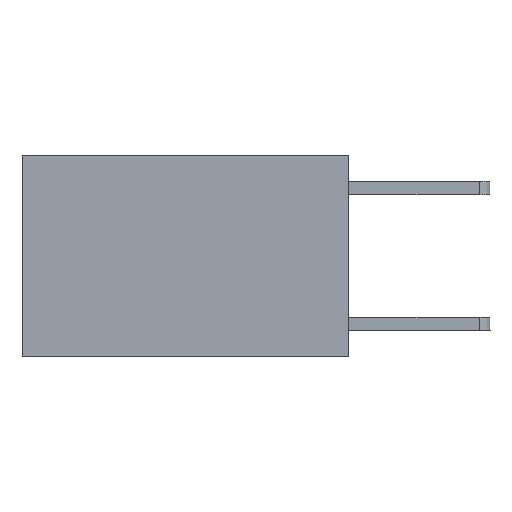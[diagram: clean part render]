
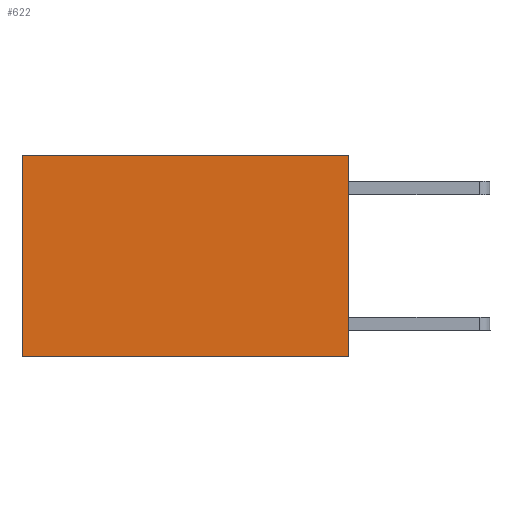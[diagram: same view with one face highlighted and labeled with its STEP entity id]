
A CAD part, left-side view. The second image highlights one B-rep face of the part: STEP entity #622.
In plain terms, the highlighted planar face has unit normal (-1, 0, 0).
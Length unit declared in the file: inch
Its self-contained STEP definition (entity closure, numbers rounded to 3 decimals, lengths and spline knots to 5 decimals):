
#97 = CARTESIAN_POINT ( 'NONE',  ( 0.2625, 0.6, -0.37 ) ) ;
#622 = ADVANCED_FACE ( 'NONE', ( #1866 ), #4625, .F. ) ;
#1021 = LINE ( 'NONE', #7380, #8252 ) ;
#1254 = VECTOR ( 'NONE', #7338, 39.37008 ) ;
#1770 = ORIENTED_EDGE ( 'NONE', *, *, #6092, .T. ) ;
#1837 = VERTEX_POINT ( 'NONE', #97 ) ;
#1866 = FACE_OUTER_BOUND ( 'NONE', #4324, .T. ) ;
#2130 = ORIENTED_EDGE ( 'NONE', *, *, #6991, .F. ) ;
#2168 = CARTESIAN_POINT ( 'NONE',  ( 0.2625, 0.6, 0. ) ) ;
#2316 = CARTESIAN_POINT ( 'NONE',  ( 0.2625, 0., -0.37 ) ) ;
#2343 = CARTESIAN_POINT ( 'NONE',  ( 0.2625, 0., -0.37 ) ) ;
#2465 = DIRECTION ( 'NONE',  ( 0., 0., -1. ) ) ;
#2494 = EDGE_CURVE ( 'NONE', #7442, #6649, #3460, .T. ) ;
#2789 = CARTESIAN_POINT ( 'NONE',  ( 0.2625, 0., 0. ) ) ;
#2866 = ORIENTED_EDGE ( 'NONE', *, *, #6940, .F. ) ;
#3460 = LINE ( 'NONE', #9207, #6965 ) ;
#4096 = ORIENTED_EDGE ( 'NONE', *, *, #2494, .T. ) ;
#4119 = DIRECTION ( 'NONE',  ( 0., 0., -1. ) ) ;
#4324 = EDGE_LOOP ( 'NONE', ( #1770, #2866, #2130, #4096 ) ) ;
#4373 = DIRECTION ( 'NONE',  ( 1., 0., 0. ) ) ;
#4475 = AXIS2_PLACEMENT_3D ( 'NONE', #5071, #4373, #4119 ) ;
#4625 = PLANE ( 'NONE',  #4475 ) ;
#5071 = CARTESIAN_POINT ( 'NONE',  ( 0.2625, 0., 0. ) ) ;
#5316 = LINE ( 'NONE', #2316, #1254 ) ;
#6092 = EDGE_CURVE ( 'NONE', #6649, #1837, #6608, .T. ) ;
#6608 = LINE ( 'NONE', #6769, #7942 ) ;
#6649 = VERTEX_POINT ( 'NONE', #2168 ) ;
#6769 = CARTESIAN_POINT ( 'NONE',  ( 0.2625, 0.6, 0. ) ) ;
#6940 = EDGE_CURVE ( 'NONE', #7828, #1837, #5316, .T. ) ;
#6965 = VECTOR ( 'NONE', #9257, 39.37008 ) ;
#6991 = EDGE_CURVE ( 'NONE', #7442, #7828, #1021, .T. ) ;
#7338 = DIRECTION ( 'NONE',  ( 0., 1., 0. ) ) ;
#7380 = CARTESIAN_POINT ( 'NONE',  ( 0.2625, 0., 0. ) ) ;
#7442 = VERTEX_POINT ( 'NONE', #2789 ) ;
#7828 = VERTEX_POINT ( 'NONE', #2343 ) ;
#7942 = VECTOR ( 'NONE', #2465, 39.37008 ) ;
#8252 = VECTOR ( 'NONE', #9292, 39.37008 ) ;
#9207 = CARTESIAN_POINT ( 'NONE',  ( 0.2625, 0., 0. ) ) ;
#9257 = DIRECTION ( 'NONE',  ( 0., 1., 0. ) ) ;
#9292 = DIRECTION ( 'NONE',  ( 0., 0., -1. ) ) ;
